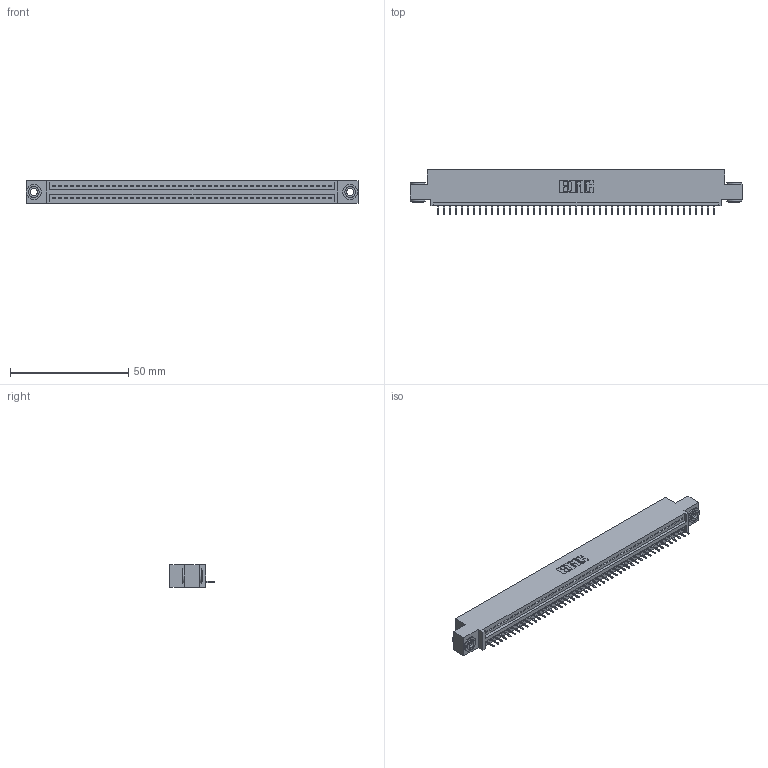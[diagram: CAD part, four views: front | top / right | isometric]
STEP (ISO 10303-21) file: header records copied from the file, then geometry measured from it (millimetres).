
FILE_DESCRIPTION (( 'STEP AP203' ), '1' );
FILE_NAME ('395-047-525-403.STEP', '2020-09-24T07:32:46', ( '' ), ( '' ), 'SwSTEP 2.0', 'SolidWorks 2020', '' );
FILE_SCHEMA (( 'CONFIG_CONTROL_DESIGN' ));
Length unit declared in the file: inch
Products named in the file (4): 345 Part_0.110 Offset - 0.156 Dia-TH; 345-292-001_345-293-125; 395-047-525-403; 345-250-002_345-250-002-102
Assembly tree (50 placements, depth 2):
  395-047-525-403
    345 Part_0.110 Offset - 0.156 Dia-TH
    345-292-001_345-293-125  x47
    345-250-002_345-250-002-102  x2
Bounding box: 140.59 x 18.72 x 9.4 mm (x, y, z)
Volume: 13148.4 mm3; surface area: 17197.4 mm2
Topology: 50 solids, 50 shells, 3082 faces, 8889 edges, 5734 vertices
Faces by surface type: plane 2256, cylinder 818, cone 8
Entity records: 35556 total; most frequent: CARTESIAN_POINT 6136, ORIENTED_EDGE 6110, DIRECTION 5383, EDGE_CURVE 3055, LINE 2715, VECTOR 2715, VERTEX_POINT 2030, AXIS2_PLACEMENT_3D 1334
